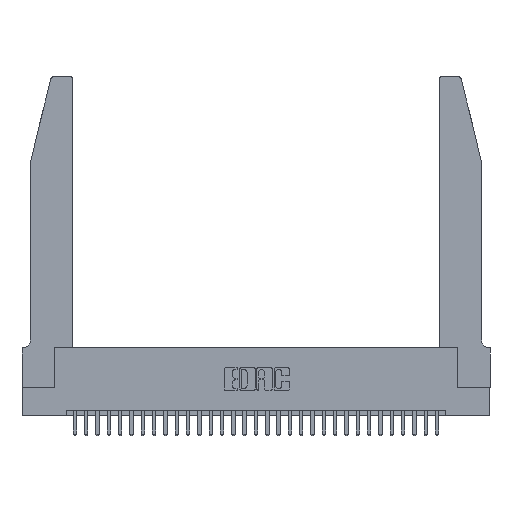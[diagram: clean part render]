
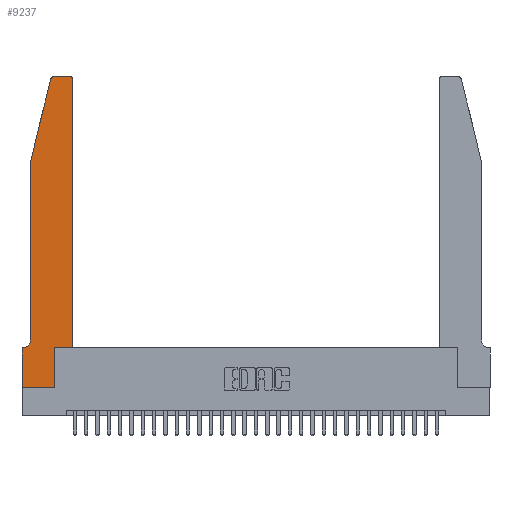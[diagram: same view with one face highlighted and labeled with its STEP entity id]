
A CAD part, top view. The second image highlights one B-rep face of the part: STEP entity #9237.
In plain terms, the highlighted planar face has unit normal (0, 0, 1).
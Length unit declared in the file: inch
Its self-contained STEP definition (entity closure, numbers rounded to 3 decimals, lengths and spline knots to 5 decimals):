
#195 = DIRECTION ( 'NONE',  ( 0., -1., 0. ) ) ;
#306 = CARTESIAN_POINT ( 'NONE',  ( 0.0755, 2., 0.37 ) ) ;
#1070 = ORIENTED_EDGE ( 'NONE', *, *, #10295, .T. ) ;
#1289 = VERTEX_POINT ( 'NONE', #20497 ) ;
#1563 = CARTESIAN_POINT ( 'NONE',  ( 0.0755, 0.42, 0.37 ) ) ;
#1840 = LINE ( 'NONE', #306, #25846 ) ;
#2954 = LINE ( 'NONE', #28014, #22017 ) ;
#4278 = CIRCLE ( 'NONE', #9339, 0.07 ) ;
#4583 = VERTEX_POINT ( 'NONE', #1563 ) ;
#5005 = ORIENTED_EDGE ( 'NONE', *, *, #29606, .T. ) ;
#5214 = VERTEX_POINT ( 'NONE', #24016 ) ;
#5656 = VERTEX_POINT ( 'NONE', #30688 ) ;
#5775 = ORIENTED_EDGE ( 'NONE', *, *, #28100, .T. ) ;
#6160 = EDGE_CURVE ( 'NONE', #17009, #5656, #24948, .T. ) ;
#6342 = VERTEX_POINT ( 'NONE', #8822 ) ;
#6721 = VECTOR ( 'NONE', #10901, 39.37008 ) ;
#7465 = VECTOR ( 'NONE', #31933, 39.37008 ) ;
#8016 = EDGE_CURVE ( 'NONE', #5214, #6342, #9211, .T. ) ;
#8044 = CARTESIAN_POINT ( 'NONE',  ( 0., 0.35, 0.37 ) ) ;
#8175 = CARTESIAN_POINT ( 'NONE',  ( 0.284, 2.72, 0.37 ) ) ;
#8361 = CARTESIAN_POINT ( 'NONE',  ( 0., 0., 0.37 ) ) ;
#8430 = VECTOR ( 'NONE', #25606, 39.37008 ) ;
#8628 = EDGE_LOOP ( 'NONE', ( #1070, #14405, #28948, #23225, #5005, #24745, #5775, #31981, #13244, #14805, #28569, #9712 ) ) ;
#8654 = EDGE_CURVE ( 'NONE', #5656, #20249, #16992, .T. ) ;
#8698 = DIRECTION ( 'NONE',  ( 0., 1., 0. ) ) ;
#8822 = CARTESIAN_POINT ( 'NONE',  ( 0.2865, 0., 0.37 ) ) ;
#9103 = DIRECTION ( 'NONE',  ( 0., 0., 1. ) ) ;
#9211 = LINE ( 'NONE', #22505, #8430 ) ;
#9237 = ADVANCED_FACE ( 'NONE', ( #14625 ), #22880, .T. ) ;
#9339 = AXIS2_PLACEMENT_3D ( 'NONE', #11331, #28492, #13836 ) ;
#9712 = ORIENTED_EDGE ( 'NONE', *, *, #10094, .T. ) ;
#9889 = VERTEX_POINT ( 'NONE', #20534 ) ;
#10094 = EDGE_CURVE ( 'NONE', #28110, #9889, #11057, .T. ) ;
#10295 = EDGE_CURVE ( 'NONE', #9889, #17009, #11439, .T. ) ;
#10578 = DIRECTION ( 'NONE',  ( 1., 0., 0. ) ) ;
#10712 = DIRECTION ( 'NONE',  ( 1., 0., 0. ) ) ;
#10901 = DIRECTION ( 'NONE',  ( 0., -1., 0. ) ) ;
#10927 = EDGE_CURVE ( 'NONE', #17293, #28110, #14135, .T. ) ;
#11012 = CARTESIAN_POINT ( 'NONE',  ( 0.284, 2.75, 0.37 ) ) ;
#11057 = CIRCLE ( 'NONE', #29488, 0.03 ) ;
#11331 = CARTESIAN_POINT ( 'NONE',  ( 0.0055, 0.42, 0.37 ) ) ;
#11439 = LINE ( 'NONE', #31974, #25283 ) ;
#13244 = ORIENTED_EDGE ( 'NONE', *, *, #23346, .T. ) ;
#13836 = DIRECTION ( 'NONE',  ( -1., 0., 0. ) ) ;
#14135 = LINE ( 'NONE', #19715, #7465 ) ;
#14173 = LINE ( 'NONE', #8361, #6721 ) ;
#14273 = EDGE_CURVE ( 'NONE', #20249, #4583, #1840, .T. ) ;
#14405 = ORIENTED_EDGE ( 'NONE', *, *, #6160, .T. ) ;
#14625 = FACE_OUTER_BOUND ( 'NONE', #8628, .T. ) ;
#14805 = ORIENTED_EDGE ( 'NONE', *, *, #21817, .T. ) ;
#15069 = CARTESIAN_POINT ( 'NONE',  ( 0.0755, 0.35, 0.37 ) ) ;
#15668 = CARTESIAN_POINT ( 'NONE',  ( 0.0755, 2., 0.37 ) ) ;
#15990 = AXIS2_PLACEMENT_3D ( 'NONE', #8044, #25328, #10578 ) ;
#16368 = CARTESIAN_POINT ( 'NONE',  ( 0.0755, 2., 0.37 ) ) ;
#16992 = LINE ( 'NONE', #15668, #29200 ) ;
#17009 = VERTEX_POINT ( 'NONE', #11012 ) ;
#17293 = VERTEX_POINT ( 'NONE', #20823 ) ;
#17384 = DIRECTION ( 'NONE',  ( -1., 0., 0. ) ) ;
#18091 = VECTOR ( 'NONE', #8698, 39.37008 ) ;
#18108 = VERTEX_POINT ( 'NONE', #26824 ) ;
#19336 = LINE ( 'NONE', #15069, #25024 ) ;
#19715 = CARTESIAN_POINT ( 'NONE',  ( 0.4505, 0.35, 0.37 ) ) ;
#20249 = VERTEX_POINT ( 'NONE', #16368 ) ;
#20497 = CARTESIAN_POINT ( 'NONE',  ( 0.0055, 0.35, 0.37 ) ) ;
#20534 = CARTESIAN_POINT ( 'NONE',  ( 0.4205, 2.75, 0.37 ) ) ;
#20823 = CARTESIAN_POINT ( 'NONE',  ( 0.4505, 0.35, 0.37 ) ) ;
#21817 = EDGE_CURVE ( 'NONE', #30710, #17293, #2954, .T. ) ;
#22017 = VECTOR ( 'NONE', #30352, 39.37008 ) ;
#22184 = EDGE_CURVE ( 'NONE', #1289, #18108, #19336, .T. ) ;
#22505 = CARTESIAN_POINT ( 'NONE',  ( 0., 0., 0.37 ) ) ;
#22880 = PLANE ( 'NONE',  #15990 ) ;
#23018 = DIRECTION ( 'NONE',  ( -0.239, -0.971, 0. ) ) ;
#23225 = ORIENTED_EDGE ( 'NONE', *, *, #14273, .T. ) ;
#23346 = EDGE_CURVE ( 'NONE', #6342, #30710, #23795, .T. ) ;
#23795 = LINE ( 'NONE', #25973, #18091 ) ;
#23897 = CARTESIAN_POINT ( 'NONE',  ( 0.4205, 2.72, 0.37 ) ) ;
#24016 = CARTESIAN_POINT ( 'NONE',  ( 0., 0., 0.37 ) ) ;
#24745 = ORIENTED_EDGE ( 'NONE', *, *, #22184, .T. ) ;
#24884 = DIRECTION ( 'NONE',  ( -1., 0., 0. ) ) ;
#24948 = CIRCLE ( 'NONE', #31254, 0.03 ) ;
#25024 = VECTOR ( 'NONE', #24884, 39.37008 ) ;
#25237 = CARTESIAN_POINT ( 'NONE',  ( 0.2865, 0.35, 0.37 ) ) ;
#25283 = VECTOR ( 'NONE', #17384, 39.37008 ) ;
#25328 = DIRECTION ( 'NONE',  ( 0., 0., 1. ) ) ;
#25457 = DIRECTION ( 'NONE',  ( 0., 0., 1. ) ) ;
#25606 = DIRECTION ( 'NONE',  ( 1., 0., 0. ) ) ;
#25631 = CARTESIAN_POINT ( 'NONE',  ( 0.4505, 2.72, 0.37 ) ) ;
#25846 = VECTOR ( 'NONE', #195, 39.37008 ) ;
#25973 = CARTESIAN_POINT ( 'NONE',  ( 0.2865, 0.35, 0.37 ) ) ;
#26359 = DIRECTION ( 'NONE',  ( 1., 0., 0. ) ) ;
#26824 = CARTESIAN_POINT ( 'NONE',  ( 0., 0.35, 0.37 ) ) ;
#28014 = CARTESIAN_POINT ( 'NONE',  ( 0.4505, 0.35, 0.37 ) ) ;
#28100 = EDGE_CURVE ( 'NONE', #18108, #5214, #14173, .T. ) ;
#28110 = VERTEX_POINT ( 'NONE', #25631 ) ;
#28492 = DIRECTION ( 'NONE',  ( 0., 0., -1. ) ) ;
#28569 = ORIENTED_EDGE ( 'NONE', *, *, #10927, .T. ) ;
#28948 = ORIENTED_EDGE ( 'NONE', *, *, #8654, .T. ) ;
#29200 = VECTOR ( 'NONE', #23018, 39.37008 ) ;
#29488 = AXIS2_PLACEMENT_3D ( 'NONE', #23897, #9103, #26359 ) ;
#29606 = EDGE_CURVE ( 'NONE', #4583, #1289, #4278, .T. ) ;
#30352 = DIRECTION ( 'NONE',  ( 1., 0., 0. ) ) ;
#30688 = CARTESIAN_POINT ( 'NONE',  ( 0.25487, 2.72718, 0.37 ) ) ;
#30710 = VERTEX_POINT ( 'NONE', #25237 ) ;
#31254 = AXIS2_PLACEMENT_3D ( 'NONE', #8175, #25457, #10712 ) ;
#31933 = DIRECTION ( 'NONE',  ( 0., 1., 0. ) ) ;
#31974 = CARTESIAN_POINT ( 'NONE',  ( 0.2605, 2.75, 0.37 ) ) ;
#31981 = ORIENTED_EDGE ( 'NONE', *, *, #8016, .T. ) ;
